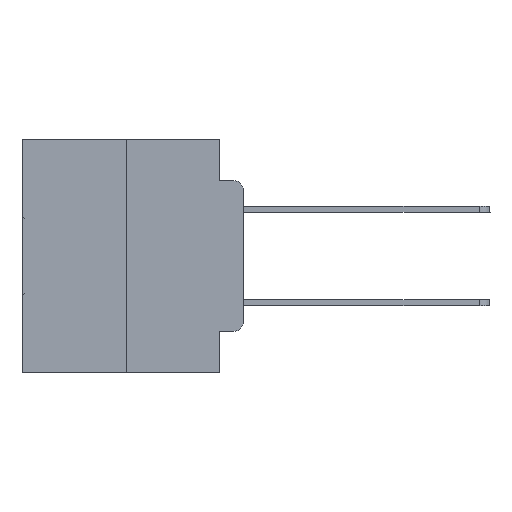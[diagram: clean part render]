
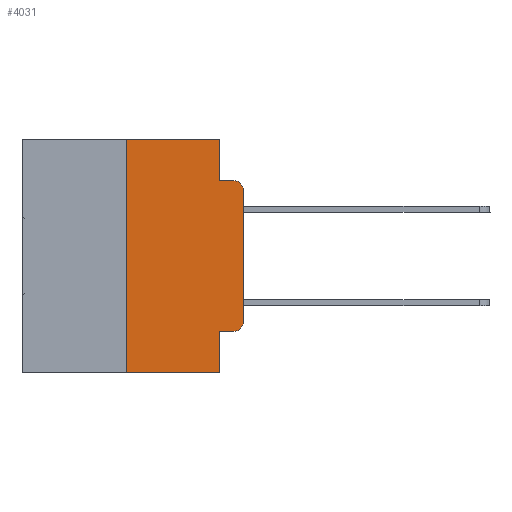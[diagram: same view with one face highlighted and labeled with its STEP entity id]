
A CAD part, left-side view. The second image highlights one B-rep face of the part: STEP entity #4031.
In plain terms, the highlighted planar face has unit normal (-1, 0, 0).
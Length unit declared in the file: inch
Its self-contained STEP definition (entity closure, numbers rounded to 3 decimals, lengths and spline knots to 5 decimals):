
#135 = DIRECTION ( 'NONE',  ( 0., -1., 0. ) ) ;
#663 = CARTESIAN_POINT ( 'NONE',  ( 0., 0., -0.3915 ) ) ;
#845 = VERTEX_POINT ( 'NONE', #9999 ) ;
#1070 = DIRECTION ( 'NONE',  ( 0., -1., 0. ) ) ;
#1483 = CARTESIAN_POINT ( 'NONE',  ( 0., 0.051, 0. ) ) ;
#1633 = DIRECTION ( 'NONE',  ( 0., 0., 1. ) ) ;
#1741 = CARTESIAN_POINT ( 'NONE',  ( 0., 0.02, -0.4115 ) ) ;
#1749 = DIRECTION ( 'NONE',  ( 1., 0., 0. ) ) ;
#2321 = ORIENTED_EDGE ( 'NONE', *, *, #22385, .F. ) ;
#3082 = DIRECTION ( 'NONE',  ( 0., 0., -1. ) ) ;
#4031 = ADVANCED_FACE ( 'NONE', ( #19952 ), #22955, .F. ) ;
#4208 = VECTOR ( 'NONE', #1633, 39.37008 ) ;
#4247 = LINE ( 'NONE', #21917, #24511 ) ;
#4426 = DIRECTION ( 'NONE',  ( 0., 0., -1. ) ) ;
#4488 = VERTEX_POINT ( 'NONE', #13363 ) ;
#4752 = VERTEX_POINT ( 'NONE', #20856 ) ;
#4910 = DIRECTION ( 'NONE',  ( 0., -1., 0. ) ) ;
#6015 = CIRCLE ( 'NONE', #16716, 0.02 ) ;
#6240 = VERTEX_POINT ( 'NONE', #663 ) ;
#6380 = CARTESIAN_POINT ( 'NONE',  ( 0., 0., 0. ) ) ;
#6549 = CARTESIAN_POINT ( 'NONE',  ( 0., 0.02, -0.3915 ) ) ;
#6965 = EDGE_CURVE ( 'NONE', #6240, #27596, #29944, .T. ) ;
#8697 = DIRECTION ( 'NONE',  ( 0., 0., 1. ) ) ;
#9067 = CARTESIAN_POINT ( 'NONE',  ( 0., 0.051, 0. ) ) ;
#9100 = VERTEX_POINT ( 'NONE', #20476 ) ;
#9989 = ORIENTED_EDGE ( 'NONE', *, *, #31066, .F. ) ;
#9999 = CARTESIAN_POINT ( 'NONE',  ( 0., 0.051, -0.0885 ) ) ;
#11032 = LINE ( 'NONE', #1483, #17747 ) ;
#11196 = EDGE_CURVE ( 'NONE', #4752, #19428, #19186, .T. ) ;
#11318 = VECTOR ( 'NONE', #135, 39.37008 ) ;
#11397 = DIRECTION ( 'NONE',  ( -1., 0., 0. ) ) ;
#11451 = VERTEX_POINT ( 'NONE', #1741 ) ;
#11468 = EDGE_CURVE ( 'NONE', #845, #28148, #19221, .T. ) ;
#12827 = CARTESIAN_POINT ( 'NONE',  ( 0., 0.473, -0.5 ) ) ;
#13089 = EDGE_CURVE ( 'NONE', #4488, #19428, #28567, .T. ) ;
#13186 = EDGE_CURVE ( 'NONE', #4488, #11451, #15691, .T. ) ;
#13363 = CARTESIAN_POINT ( 'NONE',  ( 0., 0.051, -0.4115 ) ) ;
#13402 = CARTESIAN_POINT ( 'NONE',  ( 0., 0.473, 0. ) ) ;
#13782 = DIRECTION ( 'NONE',  ( 0., 0., -1. ) ) ;
#14852 = CARTESIAN_POINT ( 'NONE',  ( 0., 0.02, -0.1085 ) ) ;
#14874 = ORIENTED_EDGE ( 'NONE', *, *, #11196, .T. ) ;
#15691 = LINE ( 'NONE', #26487, #16051 ) ;
#16051 = VECTOR ( 'NONE', #16698, 39.37008 ) ;
#16356 = VERTEX_POINT ( 'NONE', #23058 ) ;
#16698 = DIRECTION ( 'NONE',  ( 0., -1., 0. ) ) ;
#16716 = AXIS2_PLACEMENT_3D ( 'NONE', #14852, #29612, #3082 ) ;
#16746 = CARTESIAN_POINT ( 'NONE',  ( 0., 0.051, -0.0885 ) ) ;
#16944 = CARTESIAN_POINT ( 'NONE',  ( 0., 0.02, -0.0885 ) ) ;
#17144 = ORIENTED_EDGE ( 'NONE', *, *, #20251, .T. ) ;
#17747 = VECTOR ( 'NONE', #30337, 39.37008 ) ;
#17918 = CARTESIAN_POINT ( 'NONE',  ( 0., 0.051, -0.5 ) ) ;
#18031 = VECTOR ( 'NONE', #1070, 39.37008 ) ;
#18513 = LINE ( 'NONE', #25262, #4208 ) ;
#18632 = CIRCLE ( 'NONE', #19129, 0.02 ) ;
#19017 = ORIENTED_EDGE ( 'NONE', *, *, #26062, .F. ) ;
#19129 = AXIS2_PLACEMENT_3D ( 'NONE', #6549, #11397, #13782 ) ;
#19186 = LINE ( 'NONE', #12827, #18031 ) ;
#19221 = LINE ( 'NONE', #16746, #11318 ) ;
#19376 = ORIENTED_EDGE ( 'NONE', *, *, #11468, .F. ) ;
#19428 = VERTEX_POINT ( 'NONE', #17918 ) ;
#19952 = FACE_OUTER_BOUND ( 'NONE', #30062, .T. ) ;
#20251 = EDGE_CURVE ( 'NONE', #11451, #6240, #18632, .T. ) ;
#20476 = CARTESIAN_POINT ( 'NONE',  ( 0., 0.051, 0. ) ) ;
#20856 = CARTESIAN_POINT ( 'NONE',  ( 0., 0.25, -0.5 ) ) ;
#21352 = CARTESIAN_POINT ( 'NONE',  ( 0., 0., -0.1085 ) ) ;
#21917 = CARTESIAN_POINT ( 'NONE',  ( 0., 0.473, 0. ) ) ;
#22109 = VECTOR ( 'NONE', #4426, 39.37008 ) ;
#22270 = AXIS2_PLACEMENT_3D ( 'NONE', #13402, #1749, #25512 ) ;
#22385 = EDGE_CURVE ( 'NONE', #16356, #9100, #4247, .T. ) ;
#22955 = PLANE ( 'NONE',  #22270 ) ;
#23058 = CARTESIAN_POINT ( 'NONE',  ( 0., 0.25, 0. ) ) ;
#24511 = VECTOR ( 'NONE', #4910, 39.37008 ) ;
#25262 = CARTESIAN_POINT ( 'NONE',  ( 0., 0.25, 0. ) ) ;
#25512 = DIRECTION ( 'NONE',  ( 0., 0., -1. ) ) ;
#25780 = VECTOR ( 'NONE', #8697, 39.37008 ) ;
#26062 = EDGE_CURVE ( 'NONE', #9100, #845, #11032, .T. ) ;
#26091 = ORIENTED_EDGE ( 'NONE', *, *, #28294, .T. ) ;
#26487 = CARTESIAN_POINT ( 'NONE',  ( 0., 0.051, -0.4115 ) ) ;
#26953 = ORIENTED_EDGE ( 'NONE', *, *, #13089, .F. ) ;
#27134 = ORIENTED_EDGE ( 'NONE', *, *, #13186, .T. ) ;
#27596 = VERTEX_POINT ( 'NONE', #21352 ) ;
#28148 = VERTEX_POINT ( 'NONE', #16944 ) ;
#28294 = EDGE_CURVE ( 'NONE', #27596, #28148, #6015, .T. ) ;
#28567 = LINE ( 'NONE', #9067, #22109 ) ;
#29612 = DIRECTION ( 'NONE',  ( -1., 0., 0. ) ) ;
#29944 = LINE ( 'NONE', #6380, #25780 ) ;
#30062 = EDGE_LOOP ( 'NONE', ( #30325, #26091, #19376, #19017, #2321, #9989, #14874, #26953, #27134, #17144 ) ) ;
#30325 = ORIENTED_EDGE ( 'NONE', *, *, #6965, .T. ) ;
#30337 = DIRECTION ( 'NONE',  ( 0., 0., -1. ) ) ;
#31066 = EDGE_CURVE ( 'NONE', #4752, #16356, #18513, .T. ) ;
